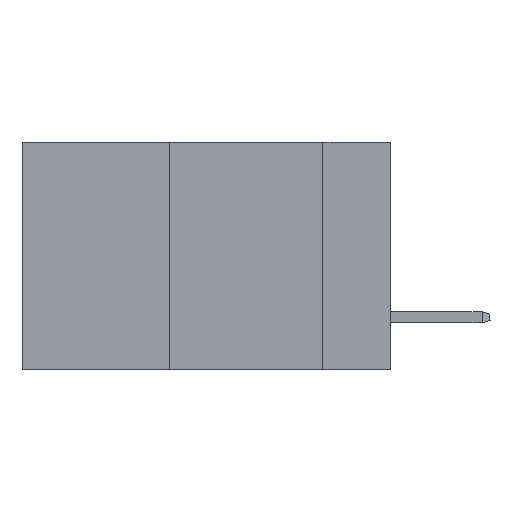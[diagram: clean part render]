
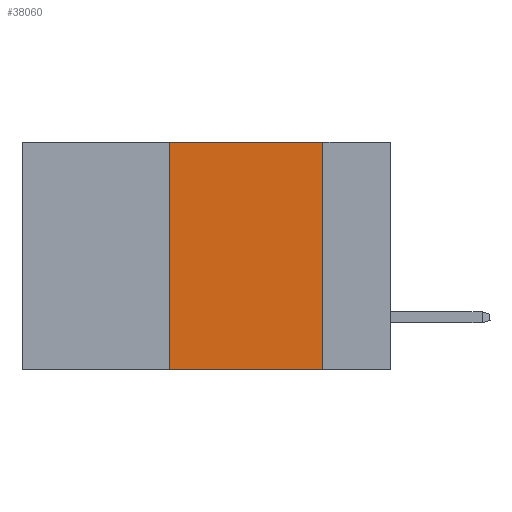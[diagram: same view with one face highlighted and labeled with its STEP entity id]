
A CAD part, left-side view. The second image highlights one B-rep face of the part: STEP entity #38060.
In plain terms, the highlighted planar face has unit normal (-1, 0, 0).
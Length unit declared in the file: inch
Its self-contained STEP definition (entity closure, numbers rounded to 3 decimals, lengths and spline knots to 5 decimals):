
#1292 = VERTEX_POINT ( 'NONE', #2738 ) ;
#1822 = EDGE_CURVE ( 'NONE', #1292, #2559, #37871, .T. ) ;
#2559 = VERTEX_POINT ( 'NONE', #7340 ) ;
#2729 = VERTEX_POINT ( 'NONE', #16843 ) ;
#2738 = CARTESIAN_POINT ( 'NONE',  ( 0., 0.36, -0.37 ) ) ;
#3246 = PLANE ( 'NONE',  #33900 ) ;
#4560 = DIRECTION ( 'NONE',  ( 0., 0., 1. ) ) ;
#5205 = ORIENTED_EDGE ( 'NONE', *, *, #7533, .T. ) ;
#5305 = DIRECTION ( 'NONE',  ( 0., -1., 0. ) ) ;
#5626 = FACE_OUTER_BOUND ( 'NONE', #38384, .T. ) ;
#7340 = CARTESIAN_POINT ( 'NONE',  ( 0., 0.36, 0. ) ) ;
#7533 = EDGE_CURVE ( 'NONE', #1292, #2729, #22009, .T. ) ;
#8207 = VECTOR ( 'NONE', #5305, 39.37008 ) ;
#8581 = CARTESIAN_POINT ( 'NONE',  ( 0., 0.6, 0. ) ) ;
#9061 = CARTESIAN_POINT ( 'NONE',  ( 0., 0.6, 0. ) ) ;
#9721 = VERTEX_POINT ( 'NONE', #34290 ) ;
#9841 = ORIENTED_EDGE ( 'NONE', *, *, #1822, .F. ) ;
#11421 = DIRECTION ( 'NONE',  ( 0., -1., 0. ) ) ;
#12174 = DIRECTION ( 'NONE',  ( 0., 0., -1. ) ) ;
#16094 = VECTOR ( 'NONE', #35918, 39.37008 ) ;
#16843 = CARTESIAN_POINT ( 'NONE',  ( 0., 0.11, -0.37 ) ) ;
#20351 = CARTESIAN_POINT ( 'NONE',  ( 0., 0.36, 0. ) ) ;
#20449 = CARTESIAN_POINT ( 'NONE',  ( 0., 0.6, -0.37 ) ) ;
#22009 = LINE ( 'NONE', #20449, #33488 ) ;
#22824 = ORIENTED_EDGE ( 'NONE', *, *, #32506, .F. ) ;
#23781 = CARTESIAN_POINT ( 'NONE',  ( 0., 0.11, 0. ) ) ;
#27521 = LINE ( 'NONE', #8581, #8207 ) ;
#30598 = DIRECTION ( 'NONE',  ( 1., 0., 0. ) ) ;
#32506 = EDGE_CURVE ( 'NONE', #9721, #2729, #38639, .T. ) ;
#33090 = VECTOR ( 'NONE', #4560, 39.37008 ) ;
#33488 = VECTOR ( 'NONE', #11421, 39.37008 ) ;
#33900 = AXIS2_PLACEMENT_3D ( 'NONE', #9061, #30598, #12174 ) ;
#34290 = CARTESIAN_POINT ( 'NONE',  ( 0., 0.11, 0. ) ) ;
#35918 = DIRECTION ( 'NONE',  ( 0., 0., -1. ) ) ;
#36325 = EDGE_CURVE ( 'NONE', #2559, #9721, #27521, .T. ) ;
#37871 = LINE ( 'NONE', #20351, #33090 ) ;
#38060 = ADVANCED_FACE ( 'NONE', ( #5626 ), #3246, .F. ) ;
#38384 = EDGE_LOOP ( 'NONE', ( #22824, #38582, #9841, #5205 ) ) ;
#38582 = ORIENTED_EDGE ( 'NONE', *, *, #36325, .F. ) ;
#38639 = LINE ( 'NONE', #23781, #16094 ) ;
